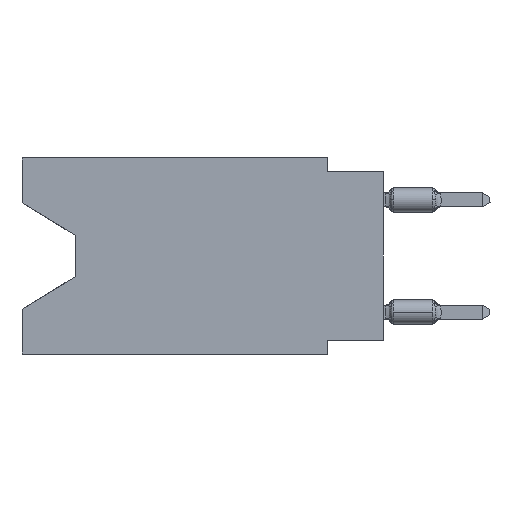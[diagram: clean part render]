
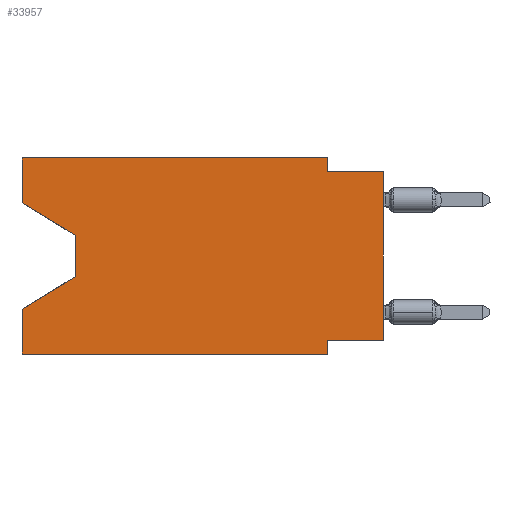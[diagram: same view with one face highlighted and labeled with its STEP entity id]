
A CAD part, left-side view. The second image highlights one B-rep face of the part: STEP entity #33957.
In plain terms, the highlighted planar face has unit normal (-1, 0, 0).
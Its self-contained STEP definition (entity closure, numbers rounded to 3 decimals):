
#303 = DIRECTION ( 'NONE',  ( 0., -0.855, -0.519 ) ) ;
#634 = CARTESIAN_POINT ( 'NONE',  ( 0., 16.383, -2.038 ) ) ;
#921 = ORIENTED_EDGE ( 'NONE', *, *, #25801, .T. ) ;
#1294 = ORIENTED_EDGE ( 'NONE', *, *, #13112, .T. ) ;
#1500 = VECTOR ( 'NONE', #11363, 1000. ) ;
#1545 = ORIENTED_EDGE ( 'NONE', *, *, #34112, .F. ) ;
#2910 = DIRECTION ( 'NONE',  ( 0., 1., 0. ) ) ;
#3062 = VECTOR ( 'NONE', #26986, 1000. ) ;
#3566 = VERTEX_POINT ( 'NONE', #15716 ) ;
#3890 = DIRECTION ( 'NONE',  ( 0., 0., -1. ) ) ;
#4582 = VECTOR ( 'NONE', #21989, 1000. ) ;
#5252 = VECTOR ( 'NONE', #18140, 1000. ) ;
#5254 = VECTOR ( 'NONE', #3890, 1000. ) ;
#5742 = CARTESIAN_POINT ( 'NONE',  ( 0., 13.97, -5.385 ) ) ;
#6041 = EDGE_CURVE ( 'NONE', #3566, #18468, #23806, .T. ) ;
#6245 = CARTESIAN_POINT ( 'NONE',  ( 0., 13.97, -5.385 ) ) ;
#6277 = VECTOR ( 'NONE', #2910, 1000. ) ;
#6415 = CARTESIAN_POINT ( 'NONE',  ( 0., 13.97, -3.505 ) ) ;
#6487 = LINE ( 'NONE', #28090, #17449 ) ;
#6818 = CARTESIAN_POINT ( 'NONE',  ( 0., 2.54, 0. ) ) ;
#7901 = EDGE_CURVE ( 'NONE', #19595, #11244, #9412, .T. ) ;
#7968 = EDGE_CURVE ( 'NONE', #29368, #24158, #33250, .T. ) ;
#8085 = LINE ( 'NONE', #634, #19741 ) ;
#8096 = VERTEX_POINT ( 'NONE', #5742 ) ;
#8215 = DIRECTION ( 'NONE',  ( 0., 0., -1. ) ) ;
#8610 = VERTEX_POINT ( 'NONE', #18597 ) ;
#8664 = AXIS2_PLACEMENT_3D ( 'NONE', #29650, #26200, #8215 ) ;
#9245 = DIRECTION ( 'NONE',  ( 0., -1., 0. ) ) ;
#9336 = CARTESIAN_POINT ( 'NONE',  ( 0., 2.54, 0. ) ) ;
#9412 = LINE ( 'NONE', #6818, #5254 ) ;
#9585 = CARTESIAN_POINT ( 'NONE',  ( 0., 16.383, 0. ) ) ;
#10318 = ORIENTED_EDGE ( 'NONE', *, *, #6041, .F. ) ;
#10669 = DIRECTION ( 'NONE',  ( 0., 0., -1. ) ) ;
#11244 = VERTEX_POINT ( 'NONE', #14117 ) ;
#11363 = DIRECTION ( 'NONE',  ( 0., 0., 1. ) ) ;
#11649 = CARTESIAN_POINT ( 'NONE',  ( 0., 0., -0.635 ) ) ;
#11702 = LINE ( 'NONE', #22241, #1500 ) ;
#12966 = DIRECTION ( 'NONE',  ( 0., 0.855, -0.519 ) ) ;
#13112 = EDGE_CURVE ( 'NONE', #3566, #17108, #24931, .T. ) ;
#13144 = CARTESIAN_POINT ( 'NONE',  ( 0., 16.383, 0. ) ) ;
#13171 = ORIENTED_EDGE ( 'NONE', *, *, #21018, .T. ) ;
#14117 = CARTESIAN_POINT ( 'NONE',  ( 0., 2.54, -0.635 ) ) ;
#14826 = VERTEX_POINT ( 'NONE', #27502 ) ;
#15112 = ORIENTED_EDGE ( 'NONE', *, *, #19616, .T. ) ;
#15716 = CARTESIAN_POINT ( 'NONE',  ( 0., 0., -8.255 ) ) ;
#16571 = CARTESIAN_POINT ( 'NONE',  ( 0., 13.97, -3.505 ) ) ;
#16633 = CARTESIAN_POINT ( 'NONE',  ( 0., 0., 0. ) ) ;
#16657 = LINE ( 'NONE', #11649, #22483 ) ;
#17108 = VERTEX_POINT ( 'NONE', #19806 ) ;
#17449 = VECTOR ( 'NONE', #9245, 1000. ) ;
#17590 = EDGE_CURVE ( 'NONE', #29368, #28825, #6487, .T. ) ;
#18102 = VECTOR ( 'NONE', #10669, 1000. ) ;
#18140 = DIRECTION ( 'NONE',  ( 0., -1., 0. ) ) ;
#18468 = VERTEX_POINT ( 'NONE', #22625 ) ;
#18597 = CARTESIAN_POINT ( 'NONE',  ( 0., 16.383, 0. ) ) ;
#18866 = EDGE_CURVE ( 'NONE', #14826, #8610, #11702, .T. ) ;
#19351 = LINE ( 'NONE', #6245, #31591 ) ;
#19595 = VERTEX_POINT ( 'NONE', #9336 ) ;
#19616 = EDGE_CURVE ( 'NONE', #22500, #8096, #27670, .T. ) ;
#19741 = VECTOR ( 'NONE', #303, 1000. ) ;
#19806 = CARTESIAN_POINT ( 'NONE',  ( 0., 0., -0.635 ) ) ;
#20030 = DIRECTION ( 'NONE',  ( 0., 0., -1. ) ) ;
#20289 = EDGE_LOOP ( 'NONE', ( #921, #15112, #13171, #21407, #21505, #31206, #10318, #1294, #1545, #22162, #31348, #31372 ) ) ;
#21018 = EDGE_CURVE ( 'NONE', #8096, #24158, #19351, .T. ) ;
#21407 = ORIENTED_EDGE ( 'NONE', *, *, #7968, .F. ) ;
#21505 = ORIENTED_EDGE ( 'NONE', *, *, #17590, .T. ) ;
#21670 = PLANE ( 'NONE',  #8664 ) ;
#21989 = DIRECTION ( 'NONE',  ( 0., 0., 1. ) ) ;
#22162 = ORIENTED_EDGE ( 'NONE', *, *, #7901, .F. ) ;
#22186 = DIRECTION ( 'NONE',  ( 0., -1., 0. ) ) ;
#22241 = CARTESIAN_POINT ( 'NONE',  ( 0., 16.383, 0. ) ) ;
#22483 = VECTOR ( 'NONE', #22186, 1000. ) ;
#22500 = VERTEX_POINT ( 'NONE', #16571 ) ;
#22625 = CARTESIAN_POINT ( 'NONE',  ( 0., 2.54, -8.255 ) ) ;
#23465 = EDGE_CURVE ( 'NONE', #8610, #19595, #23513, .T. ) ;
#23513 = LINE ( 'NONE', #13144, #5252 ) ;
#23712 = CARTESIAN_POINT ( 'NONE',  ( 0., 2.54, -8.89 ) ) ;
#23806 = LINE ( 'NONE', #25888, #6277 ) ;
#24144 = CARTESIAN_POINT ( 'NONE',  ( 0., 2.54, -8.89 ) ) ;
#24158 = VERTEX_POINT ( 'NONE', #28274 ) ;
#24931 = LINE ( 'NONE', #16633, #4582 ) ;
#25801 = EDGE_CURVE ( 'NONE', #14826, #22500, #8085, .T. ) ;
#25888 = CARTESIAN_POINT ( 'NONE',  ( 0., 0., -8.255 ) ) ;
#26200 = DIRECTION ( 'NONE',  ( 1., 0., 0. ) ) ;
#26986 = DIRECTION ( 'NONE',  ( 0., 0., 1. ) ) ;
#27502 = CARTESIAN_POINT ( 'NONE',  ( 0., 16.383, -2.038 ) ) ;
#27670 = LINE ( 'NONE', #6415, #31695 ) ;
#28090 = CARTESIAN_POINT ( 'NONE',  ( 0., 16.383, -8.89 ) ) ;
#28274 = CARTESIAN_POINT ( 'NONE',  ( 0., 16.383, -6.852 ) ) ;
#28825 = VERTEX_POINT ( 'NONE', #23712 ) ;
#29275 = EDGE_CURVE ( 'NONE', #18468, #28825, #29346, .T. ) ;
#29346 = LINE ( 'NONE', #24144, #18102 ) ;
#29368 = VERTEX_POINT ( 'NONE', #32765 ) ;
#29650 = CARTESIAN_POINT ( 'NONE',  ( 0., 16.383, 0. ) ) ;
#31206 = ORIENTED_EDGE ( 'NONE', *, *, #29275, .F. ) ;
#31348 = ORIENTED_EDGE ( 'NONE', *, *, #23465, .F. ) ;
#31372 = ORIENTED_EDGE ( 'NONE', *, *, #18866, .F. ) ;
#31591 = VECTOR ( 'NONE', #12966, 1000. ) ;
#31695 = VECTOR ( 'NONE', #20030, 1000. ) ;
#31891 = FACE_OUTER_BOUND ( 'NONE', #20289, .T. ) ;
#32765 = CARTESIAN_POINT ( 'NONE',  ( 0., 16.383, -8.89 ) ) ;
#33250 = LINE ( 'NONE', #9585, #3062 ) ;
#33957 = ADVANCED_FACE ( 'NONE', ( #31891 ), #21670, .F. ) ;
#34112 = EDGE_CURVE ( 'NONE', #11244, #17108, #16657, .T. ) ;
